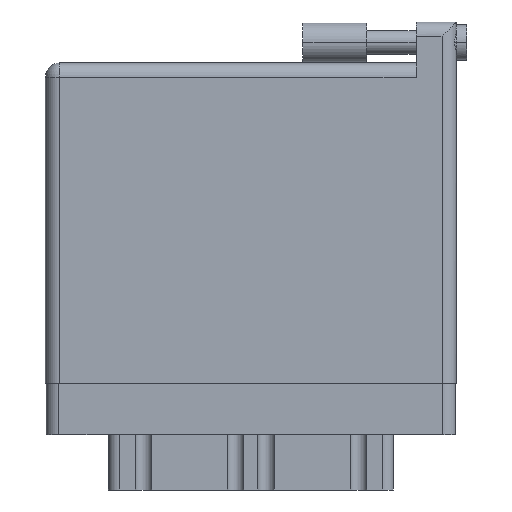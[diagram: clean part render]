
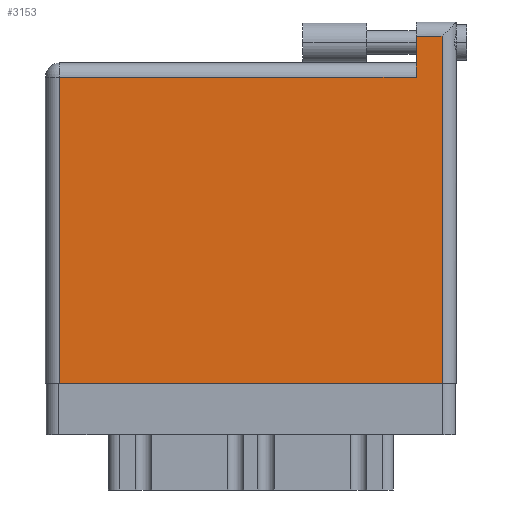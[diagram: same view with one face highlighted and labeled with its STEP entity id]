
A CAD part, front view. The second image highlights one B-rep face of the part: STEP entity #3153.
In plain terms, the highlighted face is planar.
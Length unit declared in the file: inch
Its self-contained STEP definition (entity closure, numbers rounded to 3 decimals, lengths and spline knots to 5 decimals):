
#213 = DIRECTION ( 'NONE',  ( -1., 0., 0. ) ) ;
#250 = VERTEX_POINT ( 'NONE', #508 ) ;
#508 = CARTESIAN_POINT ( 'NONE',  ( 1.811, 1.496, 0. ) ) ;
#1209 = LINE ( 'NONE', #4144, #19941 ) ;
#1517 = LINE ( 'NONE', #34043, #19492 ) ;
#2077 = VECTOR ( 'NONE', #7898, 39.37008 ) ;
#2232 = ORIENTED_EDGE ( 'NONE', *, *, #12526, .T. ) ;
#2700 = DIRECTION ( 'NONE',  ( 1., 0., 0. ) ) ;
#2946 = CARTESIAN_POINT ( 'NONE',  ( 0., 1.566, 0. ) ) ;
#3153 = ADVANCED_FACE ( 'NONE', ( #9579 ), #27112, .F. ) ;
#3325 = CARTESIAN_POINT ( 'NONE',  ( 1.811, 1.696, 0. ) ) ;
#3821 = ORIENTED_EDGE ( 'NONE', *, *, #37997, .T. ) ;
#4144 = CARTESIAN_POINT ( 'NONE',  ( 0.07, 0., 0. ) ) ;
#4163 = EDGE_CURVE ( 'NONE', #22471, #8248, #1209, .T. ) ;
#4359 = VERTEX_POINT ( 'NONE', #35123 ) ;
#6659 = DIRECTION ( 'NONE',  ( 0., -1., 0. ) ) ;
#7733 = ORIENTED_EDGE ( 'NONE', *, *, #7831, .T. ) ;
#7831 = EDGE_CURVE ( 'NONE', #250, #22471, #20444, .T. ) ;
#7898 = DIRECTION ( 'NONE',  ( 0., 1., 0. ) ) ;
#8248 = VERTEX_POINT ( 'NONE', #8697 ) ;
#8697 = CARTESIAN_POINT ( 'NONE',  ( 0.07, 0., 0. ) ) ;
#9579 = FACE_OUTER_BOUND ( 'NONE', #36068, .T. ) ;
#9724 = DIRECTION ( 'NONE',  ( -1., 0., 0. ) ) ;
#10587 = CARTESIAN_POINT ( 'NONE',  ( 1.938, 0., 0. ) ) ;
#11677 = CARTESIAN_POINT ( 'NONE',  ( 0., 0., 0. ) ) ;
#12526 = EDGE_CURVE ( 'NONE', #20202, #4359, #32250, .T. ) ;
#14620 = CARTESIAN_POINT ( 'NONE',  ( 0., 1.496, 0. ) ) ;
#14797 = EDGE_CURVE ( 'NONE', #8248, #20202, #28816, .T. ) ;
#16019 = EDGE_CURVE ( 'NONE', #25572, #250, #16743, .T. ) ;
#16229 = DIRECTION ( 'NONE',  ( 0., -1., 0. ) ) ;
#16743 = LINE ( 'NONE', #33356, #21943 ) ;
#18278 = VECTOR ( 'NONE', #32508, 39.37008 ) ;
#19492 = VECTOR ( 'NONE', #9724, 39.37008 ) ;
#19750 = ORIENTED_EDGE ( 'NONE', *, *, #16019, .T. ) ;
#19941 = VECTOR ( 'NONE', #16229, 39.37008 ) ;
#20202 = VERTEX_POINT ( 'NONE', #10587 ) ;
#20444 = LINE ( 'NONE', #14620, #18278 ) ;
#21943 = VECTOR ( 'NONE', #6659, 39.37008 ) ;
#22471 = VERTEX_POINT ( 'NONE', #36797 ) ;
#25572 = VERTEX_POINT ( 'NONE', #3325 ) ;
#26722 = DIRECTION ( 'NONE',  ( 0., 0., -1. ) ) ;
#27112 = PLANE ( 'NONE',  #28564 ) ;
#28563 = CARTESIAN_POINT ( 'NONE',  ( 1.938, 1.766, 0. ) ) ;
#28564 = AXIS2_PLACEMENT_3D ( 'NONE', #2946, #26722, #213 ) ;
#28816 = LINE ( 'NONE', #11677, #31293 ) ;
#31293 = VECTOR ( 'NONE', #2700, 39.37008 ) ;
#31618 = ORIENTED_EDGE ( 'NONE', *, *, #14797, .T. ) ;
#31914 = ORIENTED_EDGE ( 'NONE', *, *, #4163, .T. ) ;
#32250 = LINE ( 'NONE', #28563, #2077 ) ;
#32508 = DIRECTION ( 'NONE',  ( -1., 0., 0. ) ) ;
#33356 = CARTESIAN_POINT ( 'NONE',  ( 1.811, 1.766, 0. ) ) ;
#34043 = CARTESIAN_POINT ( 'NONE',  ( 0., 1.696, 0. ) ) ;
#35123 = CARTESIAN_POINT ( 'NONE',  ( 1.938, 1.696, 0. ) ) ;
#36068 = EDGE_LOOP ( 'NONE', ( #31618, #2232, #3821, #19750, #7733, #31914 ) ) ;
#36797 = CARTESIAN_POINT ( 'NONE',  ( 0.07, 1.496, 0. ) ) ;
#37997 = EDGE_CURVE ( 'NONE', #4359, #25572, #1517, .T. ) ;
